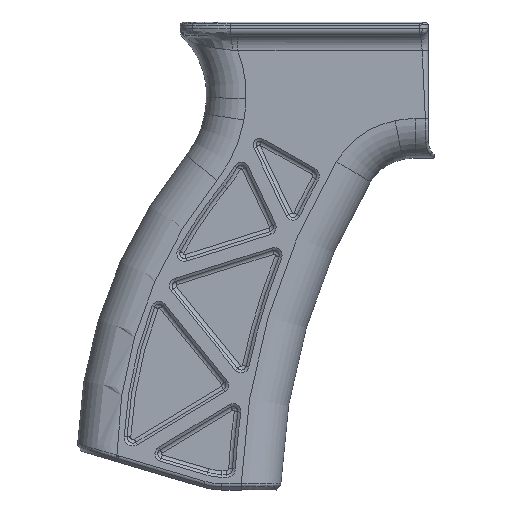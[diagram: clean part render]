
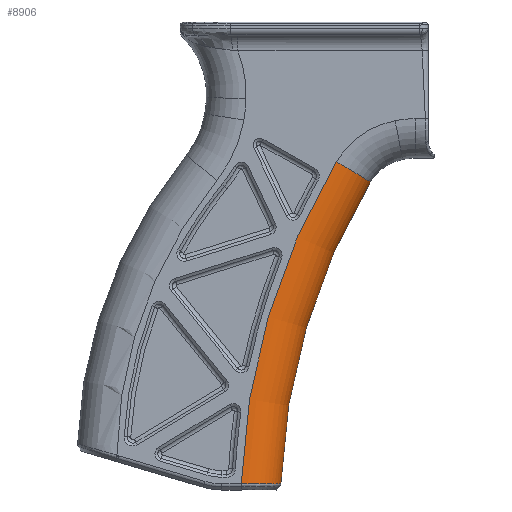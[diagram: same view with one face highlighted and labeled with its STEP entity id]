
A CAD part, front view. The second image highlights one B-rep face of the part: STEP entity #8906.
In plain terms, the highlighted toroidal (fillet/blend) face has major radius 152.175 mm and minor radius 9 mm.
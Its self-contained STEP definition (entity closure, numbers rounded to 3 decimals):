
#345=TOROIDAL_SURFACE('',#9679,152.175,9.);
#662=FACE_OUTER_BOUND('',#1267,.T.);
#1267=EDGE_LOOP('',(#6420,#6421,#6422,#6423));
#1775=B_SPLINE_CURVE_WITH_KNOTS('',3,(#13882,#13883,#13884,#13885,#13886,
#13887),.UNSPECIFIED.,.F.,.F.,(4,1,1,4),(0.,0.359,0.718,
1.257),.UNSPECIFIED.);
#2210=CIRCLE('',#9432,152.175);
#2373=CIRCLE('',#9680,143.175);
#2374=CIRCLE('',#9681,9.);
#3597=VERTEX_POINT('',#12705);
#3598=VERTEX_POINT('',#12710);
#3746=VERTEX_POINT('',#13880);
#3795=VERTEX_POINT('',#14385);
#4449=EDGE_CURVE('',#3597,#3598,#2210,.T.);
#4676=EDGE_CURVE('',#3597,#3746,#1775,.T.);
#4752=EDGE_CURVE('',#3795,#3746,#2373,.T.);
#4753=EDGE_CURVE('',#3598,#3795,#2374,.T.);
#6420=ORIENTED_EDGE('',*,*,#4449,.F.);
#6421=ORIENTED_EDGE('',*,*,#4676,.T.);
#6422=ORIENTED_EDGE('',*,*,#4752,.F.);
#6423=ORIENTED_EDGE('',*,*,#4753,.F.);
#8906=ADVANCED_FACE('',(#662),#345,.T.);
#9432=AXIS2_PLACEMENT_3D('',#12711,#10428,#10429);
#9679=AXIS2_PLACEMENT_3D('',#14384,#11015,#11016);
#9680=AXIS2_PLACEMENT_3D('',#14386,#11017,#11018);
#9681=AXIS2_PLACEMENT_3D('',#14387,#11019,#11020);
#10428=DIRECTION('center_axis',(0.,1.,0.));
#10429=DIRECTION('ref_axis',(-0.871,0.,0.491));
#11015=DIRECTION('center_axis',(0.,1.,0.));
#11016=DIRECTION('ref_axis',(0.,0.,-1.));
#11017=DIRECTION('center_axis',(0.,-1.,0.));
#11018=DIRECTION('ref_axis',(-0.871,0.,0.491));
#11019=DIRECTION('center_axis',(0.515,0.,
0.857));
#11020=DIRECTION('ref_axis',(0.,-1.,0.));
#12705=CARTESIAN_POINT('',(6.591,-10.6,-105.08));
#12710=CARTESIAN_POINT('',(28.244,-10.6,-31.771));
#12711=CARTESIAN_POINT('Origin',(158.681,-10.6,-110.152));
#13880=CARTESIAN_POINT('',(15.595,-1.6,-105.093));
#13882=CARTESIAN_POINT('Ctrl Pts',(6.591,-10.6,-105.08));
#13883=CARTESIAN_POINT('Ctrl Pts',(7.937,-10.6,-105.082));
#13884=CARTESIAN_POINT('Ctrl Pts',(10.626,-9.985,-105.085));
#13885=CARTESIAN_POINT('Ctrl Pts',(14.413,-6.975,-105.091));
#13886=CARTESIAN_POINT('Ctrl Pts',(15.595,-3.62,-105.093));
#13887=CARTESIAN_POINT('Ctrl Pts',(15.595,-1.6,-105.093));
#14384=CARTESIAN_POINT('Origin',(158.681,-1.6,-110.152));
#14385=CARTESIAN_POINT('',(35.959,-1.6,-36.407));
#14386=CARTESIAN_POINT('Origin',(158.681,-1.6,-110.152));
#14387=CARTESIAN_POINT('Origin',(28.244,-1.6,-31.771));
